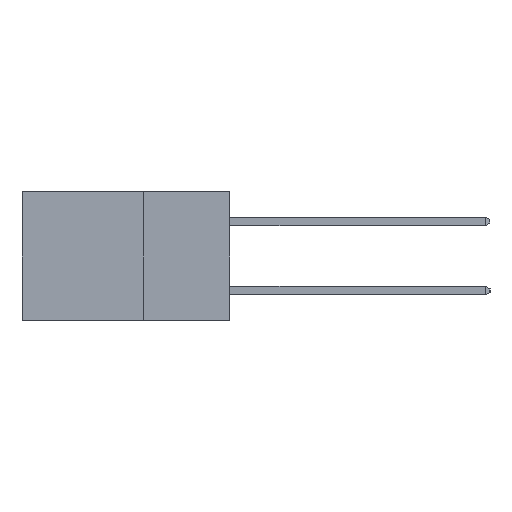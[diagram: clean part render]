
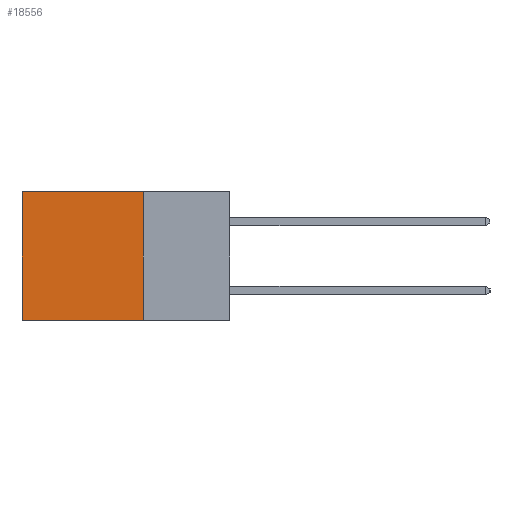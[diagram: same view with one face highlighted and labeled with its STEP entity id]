
A CAD part, left-side view. The second image highlights one B-rep face of the part: STEP entity #18556.
In plain terms, the highlighted planar face has unit normal (-1, 0, 0).
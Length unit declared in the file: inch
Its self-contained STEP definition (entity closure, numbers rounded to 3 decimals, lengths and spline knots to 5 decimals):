
#417 = CARTESIAN_POINT ( 'NONE',  ( 0.2615, 0.25, -0.37 ) ) ;
#1285 = VECTOR ( 'NONE', #13609, 39.37008 ) ;
#1452 = LINE ( 'NONE', #9649, #6373 ) ;
#1808 = LINE ( 'NONE', #5672, #1285 ) ;
#2443 = VECTOR ( 'NONE', #10618, 39.37008 ) ;
#2454 = AXIS2_PLACEMENT_3D ( 'NONE', #17583, #19159, #9720 ) ;
#2503 = CARTESIAN_POINT ( 'NONE',  ( 0.2615, 0.25, -0.37 ) ) ;
#2550 = CARTESIAN_POINT ( 'NONE',  ( 0.2615, 0.6, -0.37 ) ) ;
#3033 = LINE ( 'NONE', #417, #15372 ) ;
#3075 = ORIENTED_EDGE ( 'NONE', *, *, #7044, .F. ) ;
#3835 = FACE_OUTER_BOUND ( 'NONE', #15462, .T. ) ;
#4167 = VERTEX_POINT ( 'NONE', #9580 ) ;
#4529 = CARTESIAN_POINT ( 'NONE',  ( 0.2615, 0.25, 0. ) ) ;
#5307 = CARTESIAN_POINT ( 'NONE',  ( 0.2615, 0.6, -0.37 ) ) ;
#5522 = DIRECTION ( 'NONE',  ( 0., 1., 0. ) ) ;
#5672 = CARTESIAN_POINT ( 'NONE',  ( 0.2615, 0.25, 0. ) ) ;
#6373 = VECTOR ( 'NONE', #9603, 39.37008 ) ;
#6515 = PLANE ( 'NONE',  #2454 ) ;
#7044 = EDGE_CURVE ( 'NONE', #9855, #12680, #1452, .T. ) ;
#7331 = LINE ( 'NONE', #2550, #2443 ) ;
#9580 = CARTESIAN_POINT ( 'NONE',  ( 0.2615, 0.6, 0. ) ) ;
#9603 = DIRECTION ( 'NONE',  ( 0., 0., -1. ) ) ;
#9649 = CARTESIAN_POINT ( 'NONE',  ( 0.2615, 0.25, -0.37 ) ) ;
#9720 = DIRECTION ( 'NONE',  ( 0., 0., -1. ) ) ;
#9855 = VERTEX_POINT ( 'NONE', #4529 ) ;
#10618 = DIRECTION ( 'NONE',  ( 0., 0., -1. ) ) ;
#12680 = VERTEX_POINT ( 'NONE', #2503 ) ;
#13609 = DIRECTION ( 'NONE',  ( 0., 1., 0. ) ) ;
#15372 = VECTOR ( 'NONE', #5522, 39.37008 ) ;
#15397 = ORIENTED_EDGE ( 'NONE', *, *, #20134, .T. ) ;
#15462 = EDGE_LOOP ( 'NONE', ( #15397, #17389, #3075, #16332 ) ) ;
#16332 = ORIENTED_EDGE ( 'NONE', *, *, #17346, .T. ) ;
#17224 = VERTEX_POINT ( 'NONE', #5307 ) ;
#17346 = EDGE_CURVE ( 'NONE', #9855, #4167, #1808, .T. ) ;
#17389 = ORIENTED_EDGE ( 'NONE', *, *, #18798, .F. ) ;
#17583 = CARTESIAN_POINT ( 'NONE',  ( 0.2615, 0.25, -0.37 ) ) ;
#18556 = ADVANCED_FACE ( 'NONE', ( #3835 ), #6515, .F. ) ;
#18798 = EDGE_CURVE ( 'NONE', #12680, #17224, #3033, .T. ) ;
#19159 = DIRECTION ( 'NONE',  ( 1., 0., 0. ) ) ;
#20134 = EDGE_CURVE ( 'NONE', #4167, #17224, #7331, .T. ) ;
